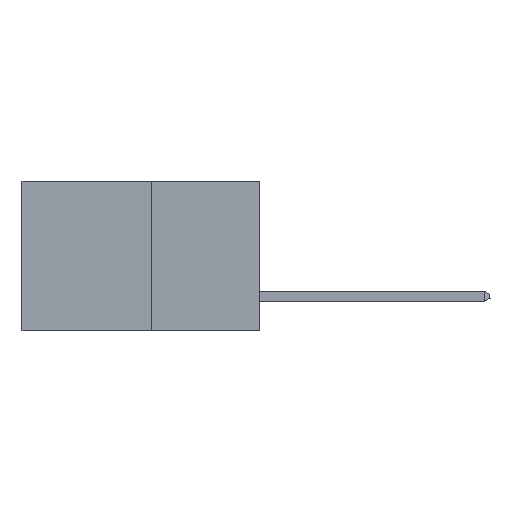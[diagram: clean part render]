
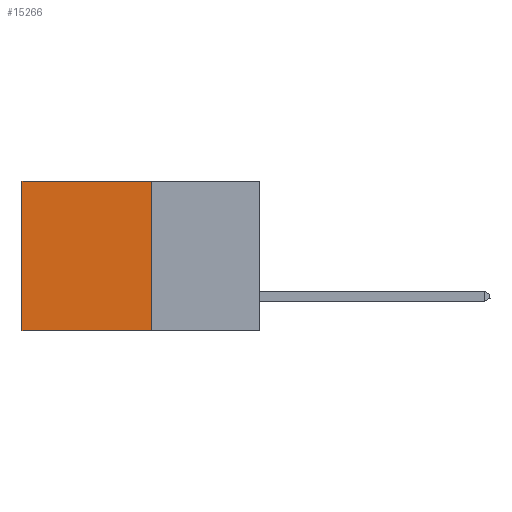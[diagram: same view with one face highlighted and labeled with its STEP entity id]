
A CAD part, left-side view. The second image highlights one B-rep face of the part: STEP entity #15266.
In plain terms, the highlighted planar face has unit normal (-1, 0, 0).
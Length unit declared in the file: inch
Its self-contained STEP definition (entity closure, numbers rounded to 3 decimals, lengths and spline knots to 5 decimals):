
#89 = CARTESIAN_POINT ( 'NONE',  ( 0.277, 0.27, -0.37 ) ) ;
#813 = FACE_OUTER_BOUND ( 'NONE', #5671, .T. ) ;
#935 = AXIS2_PLACEMENT_3D ( 'NONE', #13822, #5263, #15235 ) ;
#1010 = LINE ( 'NONE', #6256, #12129 ) ;
#1273 = CARTESIAN_POINT ( 'NONE',  ( 0.277, 0.59, -0.37 ) ) ;
#2770 = CARTESIAN_POINT ( 'NONE',  ( 0.277, 0.27, -0.37 ) ) ;
#3155 = VECTOR ( 'NONE', #11434, 39.37008 ) ;
#3536 = VECTOR ( 'NONE', #15644, 39.37008 ) ;
#3782 = PLANE ( 'NONE',  #935 ) ;
#4372 = LINE ( 'NONE', #12887, #18566 ) ;
#5263 = DIRECTION ( 'NONE',  ( 1., 0., 0. ) ) ;
#5671 = EDGE_LOOP ( 'NONE', ( #15055, #15592, #15784, #15860 ) ) ;
#6220 = EDGE_CURVE ( 'NONE', #7906, #6935, #14536, .T. ) ;
#6256 = CARTESIAN_POINT ( 'NONE',  ( 0.277, 0.27, 0. ) ) ;
#6935 = VERTEX_POINT ( 'NONE', #89 ) ;
#7464 = EDGE_CURVE ( 'NONE', #6935, #13944, #4372, .T. ) ;
#7542 = VERTEX_POINT ( 'NONE', #15920 ) ;
#7590 = CARTESIAN_POINT ( 'NONE',  ( 0.277, 0.59, -0.37 ) ) ;
#7664 = DIRECTION ( 'NONE',  ( 0., 1., 0. ) ) ;
#7906 = VERTEX_POINT ( 'NONE', #8182 ) ;
#8182 = CARTESIAN_POINT ( 'NONE',  ( 0.277, 0.27, 0. ) ) ;
#9472 = EDGE_CURVE ( 'NONE', #7542, #13944, #14623, .T. ) ;
#11434 = DIRECTION ( 'NONE',  ( 0., 0., -1. ) ) ;
#12129 = VECTOR ( 'NONE', #7664, 39.37008 ) ;
#12887 = CARTESIAN_POINT ( 'NONE',  ( 0.277, 0.27, -0.37 ) ) ;
#13822 = CARTESIAN_POINT ( 'NONE',  ( 0.277, 0.27, -0.37 ) ) ;
#13944 = VERTEX_POINT ( 'NONE', #7590 ) ;
#14322 = DIRECTION ( 'NONE',  ( 0., 1., 0. ) ) ;
#14536 = LINE ( 'NONE', #2770, #3536 ) ;
#14623 = LINE ( 'NONE', #1273, #3155 ) ;
#15055 = ORIENTED_EDGE ( 'NONE', *, *, #9472, .T. ) ;
#15235 = DIRECTION ( 'NONE',  ( 0., 0., -1. ) ) ;
#15266 = ADVANCED_FACE ( 'NONE', ( #813 ), #3782, .F. ) ;
#15592 = ORIENTED_EDGE ( 'NONE', *, *, #7464, .F. ) ;
#15644 = DIRECTION ( 'NONE',  ( 0., 0., -1. ) ) ;
#15784 = ORIENTED_EDGE ( 'NONE', *, *, #6220, .F. ) ;
#15860 = ORIENTED_EDGE ( 'NONE', *, *, #16378, .T. ) ;
#15920 = CARTESIAN_POINT ( 'NONE',  ( 0.277, 0.59, 0. ) ) ;
#16378 = EDGE_CURVE ( 'NONE', #7906, #7542, #1010, .T. ) ;
#18566 = VECTOR ( 'NONE', #14322, 39.37008 ) ;
